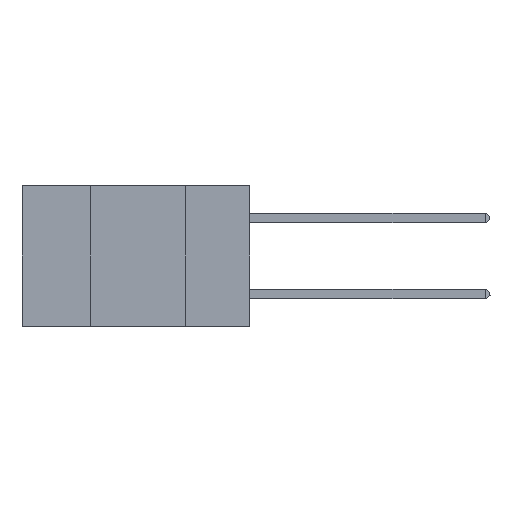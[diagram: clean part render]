
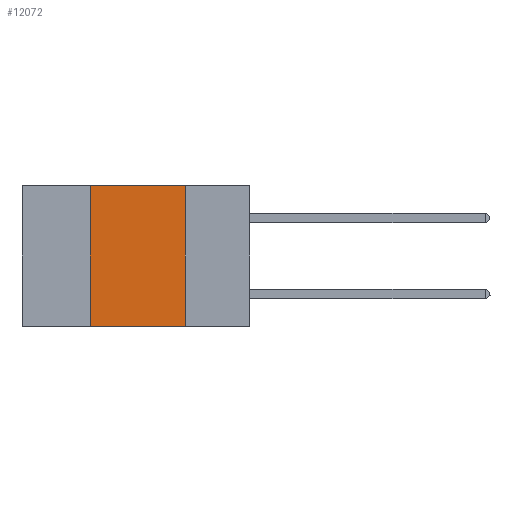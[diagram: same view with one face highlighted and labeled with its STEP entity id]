
A CAD part, left-side view. The second image highlights one B-rep face of the part: STEP entity #12072.
In plain terms, the highlighted planar face has unit normal (-1, 0, 0).
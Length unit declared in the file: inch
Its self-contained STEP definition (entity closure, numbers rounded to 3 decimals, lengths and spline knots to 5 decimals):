
#2344 = VERTEX_POINT ( 'NONE', #22775 ) ;
#2932 = CARTESIAN_POINT ( 'NONE',  ( 0., 0.17, -0.37 ) ) ;
#3385 = DIRECTION ( 'NONE',  ( 0., -1., 0. ) ) ;
#3631 = CARTESIAN_POINT ( 'NONE',  ( 0., 0.6, 0. ) ) ;
#3861 = CARTESIAN_POINT ( 'NONE',  ( 0., 0.6, 0. ) ) ;
#6609 = DIRECTION ( 'NONE',  ( 1., 0., 0. ) ) ;
#7597 = VERTEX_POINT ( 'NONE', #2932 ) ;
#8393 = LINE ( 'NONE', #3631, #9268 ) ;
#9096 = VERTEX_POINT ( 'NONE', #32103 ) ;
#9110 = VECTOR ( 'NONE', #17108, 39.37008 ) ;
#9268 = VECTOR ( 'NONE', #3385, 39.37008 ) ;
#10420 = VERTEX_POINT ( 'NONE', #32599 ) ;
#10727 = LINE ( 'NONE', #22956, #17163 ) ;
#11372 = CARTESIAN_POINT ( 'NONE',  ( 0., 0.6, -0.37 ) ) ;
#12072 = ADVANCED_FACE ( 'NONE', ( #19734 ), #31340, .F. ) ;
#13634 = EDGE_CURVE ( 'NONE', #9096, #2344, #8393, .T. ) ;
#13939 = AXIS2_PLACEMENT_3D ( 'NONE', #3861, #6609, #25924 ) ;
#16326 = EDGE_CURVE ( 'NONE', #10420, #7597, #23371, .T. ) ;
#16481 = EDGE_CURVE ( 'NONE', #10420, #9096, #26399, .T. ) ;
#17108 = DIRECTION ( 'NONE',  ( 0., -1., 0. ) ) ;
#17163 = VECTOR ( 'NONE', #19698, 39.37008 ) ;
#19698 = DIRECTION ( 'NONE',  ( 0., 0., -1. ) ) ;
#19734 = FACE_OUTER_BOUND ( 'NONE', #31624, .T. ) ;
#21274 = CARTESIAN_POINT ( 'NONE',  ( 0., 0.42, 0. ) ) ;
#22775 = CARTESIAN_POINT ( 'NONE',  ( 0., 0.17, 0. ) ) ;
#22956 = CARTESIAN_POINT ( 'NONE',  ( 0., 0.17, 0. ) ) ;
#23371 = LINE ( 'NONE', #11372, #9110 ) ;
#25834 = ORIENTED_EDGE ( 'NONE', *, *, #13634, .F. ) ;
#25924 = DIRECTION ( 'NONE',  ( 0., 0., -1. ) ) ;
#26399 = LINE ( 'NONE', #21274, #34581 ) ;
#27231 = ORIENTED_EDGE ( 'NONE', *, *, #16326, .T. ) ;
#27490 = ORIENTED_EDGE ( 'NONE', *, *, #30417, .F. ) ;
#30417 = EDGE_CURVE ( 'NONE', #2344, #7597, #10727, .T. ) ;
#31340 = PLANE ( 'NONE',  #13939 ) ;
#31624 = EDGE_LOOP ( 'NONE', ( #27490, #25834, #35323, #27231 ) ) ;
#32103 = CARTESIAN_POINT ( 'NONE',  ( 0., 0.42, 0. ) ) ;
#32599 = CARTESIAN_POINT ( 'NONE',  ( 0., 0.42, -0.37 ) ) ;
#34581 = VECTOR ( 'NONE', #35382, 39.37008 ) ;
#35323 = ORIENTED_EDGE ( 'NONE', *, *, #16481, .F. ) ;
#35382 = DIRECTION ( 'NONE',  ( 0., 0., 1. ) ) ;
